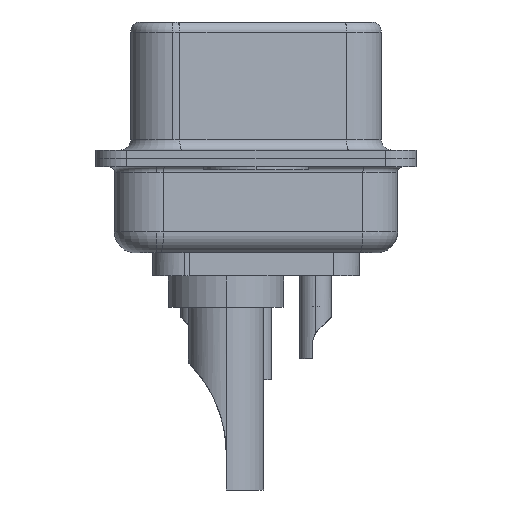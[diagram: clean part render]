
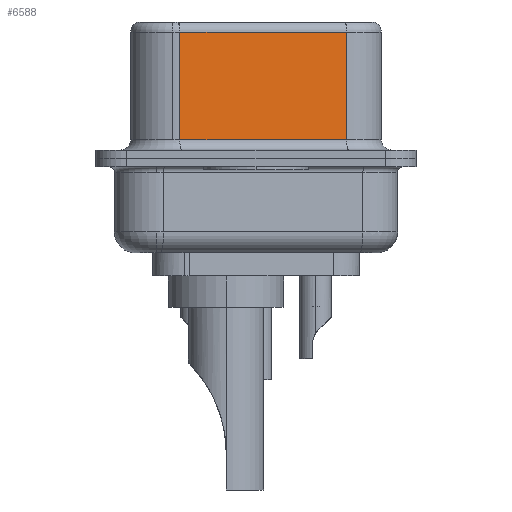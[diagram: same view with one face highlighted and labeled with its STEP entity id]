
A CAD part, left-side view. The second image highlights one B-rep face of the part: STEP entity #6588.
In plain terms, the highlighted planar face has unit normal (-0.985, -0.174, 0).
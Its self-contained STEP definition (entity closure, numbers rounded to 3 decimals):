
#450 = LINE ( 'NONE', #6074, #5079 ) ;
#735 = VERTEX_POINT ( 'NONE', #18851 ) ;
#1604 = CARTESIAN_POINT ( 'NONE',  ( 5.132, -4.322, 0.9 ) ) ;
#1899 = ORIENTED_EDGE ( 'NONE', *, *, #8309, .T. ) ;
#3764 = PLANE ( 'NONE',  #7904 ) ;
#4012 = ORIENTED_EDGE ( 'NONE', *, *, #16339, .T. ) ;
#5079 = VECTOR ( 'NONE', #8999, 1000. ) ;
#5215 = DIRECTION ( 'NONE',  ( 0., 0., -1. ) ) ;
#5259 = LINE ( 'NONE', #20524, #15641 ) ;
#5909 = EDGE_CURVE ( 'NONE', #23757, #19311, #450, .T. ) ;
#6074 = CARTESIAN_POINT ( 'NONE',  ( 5.132, -4.322, 6.02 ) ) ;
#6588 = ADVANCED_FACE ( 'NONE', ( #12416 ), #3764, .F. ) ;
#6704 = DIRECTION ( 'NONE',  ( 0., 0., -1. ) ) ;
#7306 = EDGE_CURVE ( 'NONE', #23757, #23592, #8359, .T. ) ;
#7904 = AXIS2_PLACEMENT_3D ( 'NONE', #13621, #17791, #18149 ) ;
#8309 = EDGE_CURVE ( 'NONE', #19311, #735, #5259, .T. ) ;
#8359 = LINE ( 'NONE', #24214, #17944 ) ;
#8999 = DIRECTION ( 'NONE',  ( -0.174, 0.985, 0. ) ) ;
#12052 = ORIENTED_EDGE ( 'NONE', *, *, #7306, .F. ) ;
#12416 = FACE_OUTER_BOUND ( 'NONE', #19869, .T. ) ;
#13325 = DIRECTION ( 'NONE',  ( 0.174, -0.985, 0. ) ) ;
#13621 = CARTESIAN_POINT ( 'NONE',  ( 5.132, -4.322, 6.52 ) ) ;
#13639 = LINE ( 'NONE', #1604, #18036 ) ;
#15641 = VECTOR ( 'NONE', #5215, 1000. ) ;
#16339 = EDGE_CURVE ( 'NONE', #735, #23592, #13639, .T. ) ;
#17404 = CARTESIAN_POINT ( 'NONE',  ( 5.132, -4.322, 0.9 ) ) ;
#17791 = DIRECTION ( 'NONE',  ( 0.985, 0.174, 0. ) ) ;
#17832 = ORIENTED_EDGE ( 'NONE', *, *, #5909, .T. ) ;
#17944 = VECTOR ( 'NONE', #6704, 1000. ) ;
#18036 = VECTOR ( 'NONE', #13325, 1000. ) ;
#18149 = DIRECTION ( 'NONE',  ( -0.174, 0.985, 0. ) ) ;
#18851 = CARTESIAN_POINT ( 'NONE',  ( 3.73, 3.628, 0.9 ) ) ;
#19311 = VERTEX_POINT ( 'NONE', #24135 ) ;
#19869 = EDGE_LOOP ( 'NONE', ( #12052, #17832, #1899, #4012 ) ) ;
#20524 = CARTESIAN_POINT ( 'NONE',  ( 3.73, 3.628, 6.52 ) ) ;
#23582 = CARTESIAN_POINT ( 'NONE',  ( 5.132, -4.322, 6.02 ) ) ;
#23592 = VERTEX_POINT ( 'NONE', #17404 ) ;
#23757 = VERTEX_POINT ( 'NONE', #23582 ) ;
#24135 = CARTESIAN_POINT ( 'NONE',  ( 3.73, 3.628, 6.02 ) ) ;
#24214 = CARTESIAN_POINT ( 'NONE',  ( 5.132, -4.322, 6.52 ) ) ;
